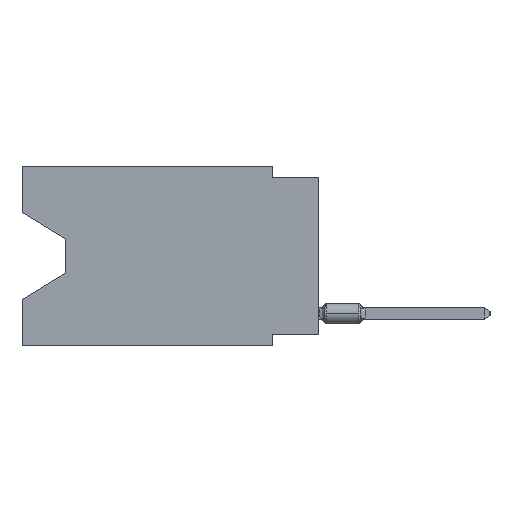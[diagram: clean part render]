
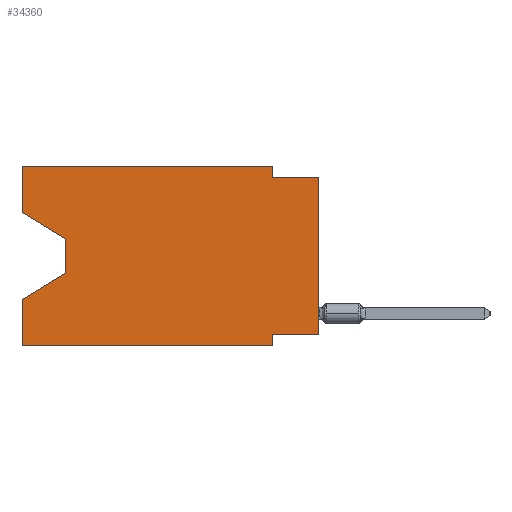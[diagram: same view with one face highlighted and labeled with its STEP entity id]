
A CAD part, left-side view. The second image highlights one B-rep face of the part: STEP entity #34360.
In plain terms, the highlighted planar face has unit normal (-1, 0, 0).
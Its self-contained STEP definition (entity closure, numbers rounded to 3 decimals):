
#49 = EDGE_CURVE ( 'NONE', #19654, #12369, #612, .T. ) ;
#77 = DIRECTION ( 'NONE',  ( 0., -1., 0. ) ) ;
#340 = VECTOR ( 'NONE', #33598, 1000. ) ;
#612 = LINE ( 'NONE', #24138, #20992 ) ;
#1229 = ORIENTED_EDGE ( 'NONE', *, *, #26193, .F. ) ;
#1272 = LINE ( 'NONE', #11996, #6490 ) ;
#1381 = CARTESIAN_POINT ( 'NONE',  ( 0., 2.54, -0.635 ) ) ;
#1656 = CARTESIAN_POINT ( 'NONE',  ( 0., 16.383, 0. ) ) ;
#2362 = VERTEX_POINT ( 'NONE', #17177 ) ;
#2891 = VERTEX_POINT ( 'NONE', #29290 ) ;
#3277 = EDGE_CURVE ( 'NONE', #6477, #2891, #32044, .T. ) ;
#3292 = CARTESIAN_POINT ( 'NONE',  ( 0., 13.97, -5.893 ) ) ;
#3335 = ORIENTED_EDGE ( 'NONE', *, *, #29991, .F. ) ;
#3457 = EDGE_CURVE ( 'NONE', #5456, #11497, #13470, .T. ) ;
#3773 = ORIENTED_EDGE ( 'NONE', *, *, #14282, .F. ) ;
#4039 = VECTOR ( 'NONE', #16214, 1000. ) ;
#4568 = VECTOR ( 'NONE', #14139, 1000. ) ;
#4578 = ORIENTED_EDGE ( 'NONE', *, *, #20328, .T. ) ;
#4978 = LINE ( 'NONE', #1656, #22404 ) ;
#5308 = CARTESIAN_POINT ( 'NONE',  ( 0., 13.97, -4.013 ) ) ;
#5456 = VERTEX_POINT ( 'NONE', #14461 ) ;
#5458 = PLANE ( 'NONE',  #26546 ) ;
#6477 = VERTEX_POINT ( 'NONE', #30331 ) ;
#6490 = VECTOR ( 'NONE', #33739, 1000. ) ;
#6965 = ORIENTED_EDGE ( 'NONE', *, *, #3457, .T. ) ;
#7534 = CARTESIAN_POINT ( 'NONE',  ( 0., 16.383, 0. ) ) ;
#7593 = DIRECTION ( 'NONE',  ( 1., 0., 0. ) ) ;
#8002 = EDGE_LOOP ( 'NONE', ( #4578, #15491, #6965, #3773, #15462, #1229, #11432, #23033, #33379, #3335, #30941, #32010 ) ) ;
#8106 = FACE_OUTER_BOUND ( 'NONE', #8002, .T. ) ;
#8339 = EDGE_CURVE ( 'NONE', #2362, #13500, #1272, .T. ) ;
#9283 = LINE ( 'NONE', #24861, #18473 ) ;
#10001 = DIRECTION ( 'NONE',  ( 0., 0., 1. ) ) ;
#11432 = ORIENTED_EDGE ( 'NONE', *, *, #8339, .F. ) ;
#11497 = VERTEX_POINT ( 'NONE', #13890 ) ;
#11996 = CARTESIAN_POINT ( 'NONE',  ( 0., 0., -9.271 ) ) ;
#12046 = LINE ( 'NONE', #20266, #4568 ) ;
#12369 = VERTEX_POINT ( 'NONE', #33094 ) ;
#12472 = LINE ( 'NONE', #23158, #31019 ) ;
#12642 = CARTESIAN_POINT ( 'NONE',  ( 0., 2.54, -9.271 ) ) ;
#13274 = VECTOR ( 'NONE', #23206, 1000. ) ;
#13470 = LINE ( 'NONE', #3292, #32114 ) ;
#13500 = VERTEX_POINT ( 'NONE', #12642 ) ;
#13540 = EDGE_CURVE ( 'NONE', #34703, #24705, #12472, .T. ) ;
#13662 = LINE ( 'NONE', #27163, #340 ) ;
#13890 = CARTESIAN_POINT ( 'NONE',  ( 0., 16.383, -7.36 ) ) ;
#14139 = DIRECTION ( 'NONE',  ( 0., 0., -1. ) ) ;
#14282 = EDGE_CURVE ( 'NONE', #34703, #11497, #4978, .T. ) ;
#14461 = CARTESIAN_POINT ( 'NONE',  ( 0., 13.97, -5.893 ) ) ;
#15313 = VECTOR ( 'NONE', #10001, 1000. ) ;
#15392 = EDGE_CURVE ( 'NONE', #17557, #5456, #12046, .T. ) ;
#15462 = ORIENTED_EDGE ( 'NONE', *, *, #13540, .T. ) ;
#15491 = ORIENTED_EDGE ( 'NONE', *, *, #15392, .T. ) ;
#15642 = CARTESIAN_POINT ( 'NONE',  ( 0., 16.383, 0. ) ) ;
#15678 = DIRECTION ( 'NONE',  ( 0., 0., 1. ) ) ;
#15778 = LINE ( 'NONE', #32435, #23673 ) ;
#16160 = DIRECTION ( 'NONE',  ( 0., 0., -1. ) ) ;
#16214 = DIRECTION ( 'NONE',  ( 0., 0., -1. ) ) ;
#16420 = EDGE_CURVE ( 'NONE', #2362, #12369, #9283, .T. ) ;
#17177 = CARTESIAN_POINT ( 'NONE',  ( 0., 0., -9.271 ) ) ;
#17557 = VERTEX_POINT ( 'NONE', #5308 ) ;
#18473 = VECTOR ( 'NONE', #32936, 1000. ) ;
#19654 = VERTEX_POINT ( 'NONE', #1381 ) ;
#20266 = CARTESIAN_POINT ( 'NONE',  ( 0., 13.97, -4.013 ) ) ;
#20328 = EDGE_CURVE ( 'NONE', #6477, #17557, #15778, .T. ) ;
#20992 = VECTOR ( 'NONE', #77, 1000. ) ;
#21522 = DIRECTION ( 'NONE',  ( 0., 0.855, -0.519 ) ) ;
#22404 = VECTOR ( 'NONE', #15678, 1000. ) ;
#22811 = VERTEX_POINT ( 'NONE', #26672 ) ;
#23033 = ORIENTED_EDGE ( 'NONE', *, *, #16420, .T. ) ;
#23158 = CARTESIAN_POINT ( 'NONE',  ( 0., 16.383, -9.906 ) ) ;
#23206 = DIRECTION ( 'NONE',  ( 0., -1., 0. ) ) ;
#23583 = LINE ( 'NONE', #31831, #4039 ) ;
#23673 = VECTOR ( 'NONE', #34564, 1000. ) ;
#24138 = CARTESIAN_POINT ( 'NONE',  ( 0., 0., -0.635 ) ) ;
#24705 = VERTEX_POINT ( 'NONE', #28006 ) ;
#24861 = CARTESIAN_POINT ( 'NONE',  ( 0., 0., 0. ) ) ;
#26174 = CARTESIAN_POINT ( 'NONE',  ( 0., 16.383, 0. ) ) ;
#26193 = EDGE_CURVE ( 'NONE', #13500, #24705, #13662, .T. ) ;
#26546 = AXIS2_PLACEMENT_3D ( 'NONE', #15642, #7593, #16160 ) ;
#26672 = CARTESIAN_POINT ( 'NONE',  ( 0., 2.54, 0. ) ) ;
#26714 = EDGE_CURVE ( 'NONE', #2891, #22811, #33731, .T. ) ;
#27163 = CARTESIAN_POINT ( 'NONE',  ( 0., 2.54, -9.906 ) ) ;
#28006 = CARTESIAN_POINT ( 'NONE',  ( 0., 2.54, -9.906 ) ) ;
#29290 = CARTESIAN_POINT ( 'NONE',  ( 0., 16.383, 0. ) ) ;
#29991 = EDGE_CURVE ( 'NONE', #22811, #19654, #23583, .T. ) ;
#30331 = CARTESIAN_POINT ( 'NONE',  ( 0., 16.383, -2.546 ) ) ;
#30941 = ORIENTED_EDGE ( 'NONE', *, *, #26714, .F. ) ;
#31019 = VECTOR ( 'NONE', #33865, 1000. ) ;
#31831 = CARTESIAN_POINT ( 'NONE',  ( 0., 2.54, 0. ) ) ;
#32010 = ORIENTED_EDGE ( 'NONE', *, *, #3277, .F. ) ;
#32044 = LINE ( 'NONE', #7534, #15313 ) ;
#32114 = VECTOR ( 'NONE', #21522, 1000. ) ;
#32378 = CARTESIAN_POINT ( 'NONE',  ( 0., 16.383, -9.906 ) ) ;
#32435 = CARTESIAN_POINT ( 'NONE',  ( 0., 16.383, -2.546 ) ) ;
#32936 = DIRECTION ( 'NONE',  ( 0., 0., 1. ) ) ;
#33094 = CARTESIAN_POINT ( 'NONE',  ( 0., 0., -0.635 ) ) ;
#33379 = ORIENTED_EDGE ( 'NONE', *, *, #49, .F. ) ;
#33598 = DIRECTION ( 'NONE',  ( 0., 0., -1. ) ) ;
#33731 = LINE ( 'NONE', #26174, #13274 ) ;
#33739 = DIRECTION ( 'NONE',  ( 0., 1., 0. ) ) ;
#33865 = DIRECTION ( 'NONE',  ( 0., -1., 0. ) ) ;
#34360 = ADVANCED_FACE ( 'NONE', ( #8106 ), #5458, .F. ) ;
#34564 = DIRECTION ( 'NONE',  ( 0., -0.855, -0.519 ) ) ;
#34703 = VERTEX_POINT ( 'NONE', #32378 ) ;
